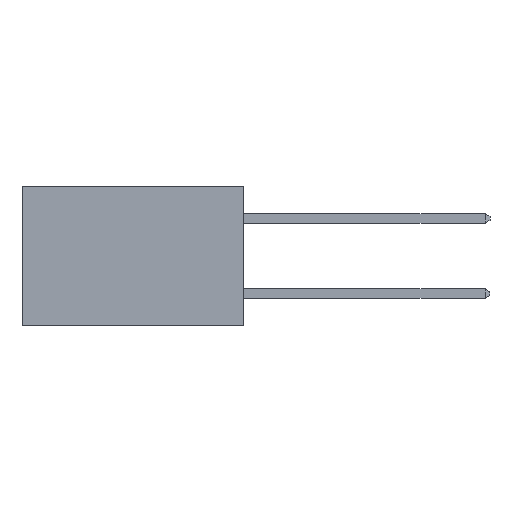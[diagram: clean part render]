
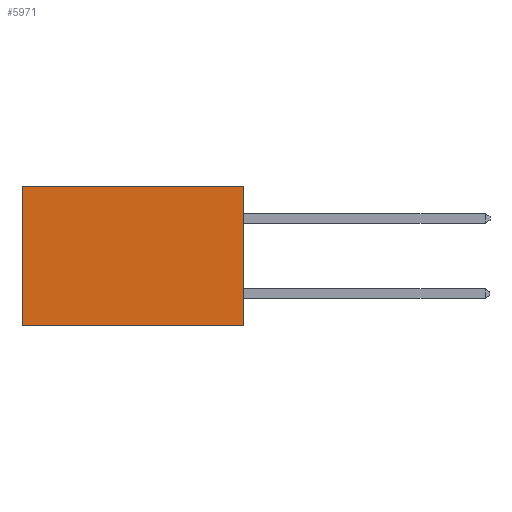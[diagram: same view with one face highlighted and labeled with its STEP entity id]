
A CAD part, left-side view. The second image highlights one B-rep face of the part: STEP entity #5971.
In plain terms, the highlighted planar face has unit normal (-1, 0, 0).
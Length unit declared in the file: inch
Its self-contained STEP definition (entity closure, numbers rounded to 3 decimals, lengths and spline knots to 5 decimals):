
#436 = EDGE_CURVE ( 'NONE', #5734, #6417, #3946, .T. ) ;
#456 = EDGE_CURVE ( 'NONE', #7914, #5734, #5636, .T. ) ;
#786 = VECTOR ( 'NONE', #5948, 39.37008 ) ;
#880 = EDGE_LOOP ( 'NONE', ( #8733, #8992, #10225, #1354 ) ) ;
#916 = EDGE_CURVE ( 'NONE', #8318, #6417, #9527, .T. ) ;
#1354 = ORIENTED_EDGE ( 'NONE', *, *, #8805, .T. ) ;
#2769 = VECTOR ( 'NONE', #8468, 39.37008 ) ;
#3543 = CARTESIAN_POINT ( 'NONE',  ( 0.277, 0.59, -0.37 ) ) ;
#3946 = LINE ( 'NONE', #9024, #8157 ) ;
#4092 = CARTESIAN_POINT ( 'NONE',  ( 0.277, 0.59, -0.37 ) ) ;
#5223 = FACE_OUTER_BOUND ( 'NONE', #880, .T. ) ;
#5332 = CARTESIAN_POINT ( 'NONE',  ( 0.277, 0., 0. ) ) ;
#5636 = LINE ( 'NONE', #5667, #786 ) ;
#5667 = CARTESIAN_POINT ( 'NONE',  ( 0.277, 0., -0.37 ) ) ;
#5734 = VERTEX_POINT ( 'NONE', #8987 ) ;
#5948 = DIRECTION ( 'NONE',  ( 0., 0., -1. ) ) ;
#5971 = ADVANCED_FACE ( 'NONE', ( #5223 ), #7352, .F. ) ;
#6417 = VERTEX_POINT ( 'NONE', #4092 ) ;
#7303 = DIRECTION ( 'NONE',  ( 0., 0., -1. ) ) ;
#7341 = DIRECTION ( 'NONE',  ( 1., 0., 0. ) ) ;
#7352 = PLANE ( 'NONE',  #8792 ) ;
#7871 = CARTESIAN_POINT ( 'NONE',  ( 0.277, 0., -0.37 ) ) ;
#7892 = CARTESIAN_POINT ( 'NONE',  ( 0.277, 0., 0. ) ) ;
#7914 = VERTEX_POINT ( 'NONE', #5332 ) ;
#8157 = VECTOR ( 'NONE', #8879, 39.37008 ) ;
#8318 = VERTEX_POINT ( 'NONE', #9808 ) ;
#8468 = DIRECTION ( 'NONE',  ( 0., 0., -1. ) ) ;
#8733 = ORIENTED_EDGE ( 'NONE', *, *, #916, .T. ) ;
#8792 = AXIS2_PLACEMENT_3D ( 'NONE', #7871, #7341, #7303 ) ;
#8805 = EDGE_CURVE ( 'NONE', #7914, #8318, #10747, .T. ) ;
#8879 = DIRECTION ( 'NONE',  ( 0., 1., 0. ) ) ;
#8987 = CARTESIAN_POINT ( 'NONE',  ( 0.277, 0., -0.37 ) ) ;
#8992 = ORIENTED_EDGE ( 'NONE', *, *, #436, .F. ) ;
#9024 = CARTESIAN_POINT ( 'NONE',  ( 0.277, 0., -0.37 ) ) ;
#9527 = LINE ( 'NONE', #3543, #2769 ) ;
#9771 = VECTOR ( 'NONE', #11046, 39.37008 ) ;
#9808 = CARTESIAN_POINT ( 'NONE',  ( 0.277, 0.59, 0. ) ) ;
#10225 = ORIENTED_EDGE ( 'NONE', *, *, #456, .F. ) ;
#10747 = LINE ( 'NONE', #7892, #9771 ) ;
#11046 = DIRECTION ( 'NONE',  ( 0., 1., 0. ) ) ;
